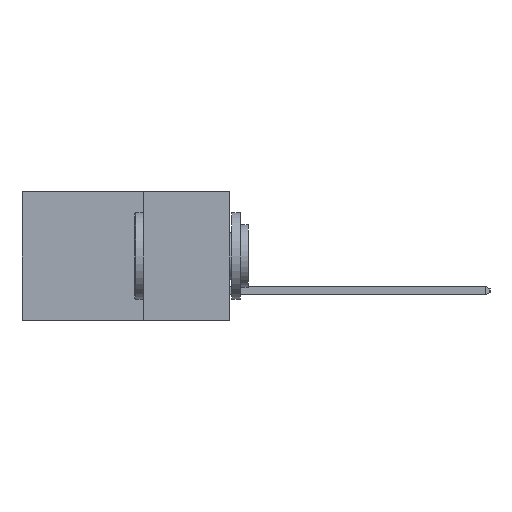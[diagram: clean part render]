
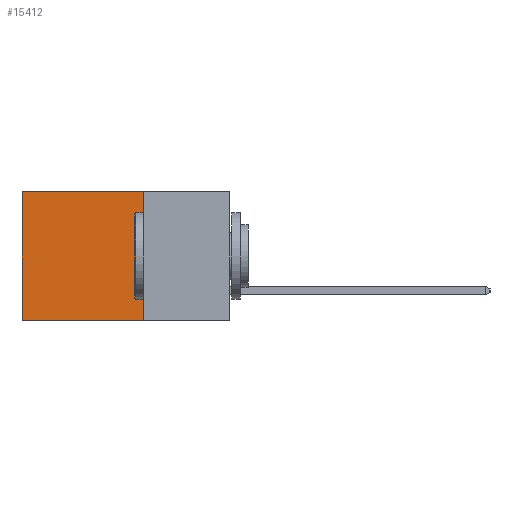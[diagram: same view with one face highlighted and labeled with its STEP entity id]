
A CAD part, left-side view. The second image highlights one B-rep face of the part: STEP entity #15412.
In plain terms, the highlighted planar face has unit normal (-1, 0, 0).
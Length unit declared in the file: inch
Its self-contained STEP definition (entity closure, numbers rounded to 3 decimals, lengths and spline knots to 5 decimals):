
#64 = VECTOR ( 'NONE', #19857, 39.37008 ) ;
#353 = DIRECTION ( 'NONE',  ( 0., 0., -1. ) ) ;
#356 = DIRECTION ( 'NONE',  ( 1., 0., 0. ) ) ;
#441 = PLANE ( 'NONE',  #8171 ) ;
#489 = CARTESIAN_POINT ( 'NONE',  ( 0.2615, 0.25, -0.37 ) ) ;
#1026 = ORIENTED_EDGE ( 'NONE', *, *, #11338, .T. ) ;
#1472 = LINE ( 'NONE', #2624, #6753 ) ;
#2441 = DIRECTION ( 'NONE',  ( 0., 0., -1. ) ) ;
#2473 = ORIENTED_EDGE ( 'NONE', *, *, #11125, .F. ) ;
#2490 = DIRECTION ( 'NONE',  ( 0., 1., 0. ) ) ;
#2624 = CARTESIAN_POINT ( 'NONE',  ( 0.2615, 0.6, -0.37 ) ) ;
#4432 = VERTEX_POINT ( 'NONE', #12737 ) ;
#5304 = EDGE_LOOP ( 'NONE', ( #17439, #21790, #2473, #1026 ) ) ;
#5968 = VERTEX_POINT ( 'NONE', #16197 ) ;
#6753 = VECTOR ( 'NONE', #2441, 39.37008 ) ;
#7382 = VERTEX_POINT ( 'NONE', #9404 ) ;
#8124 = CARTESIAN_POINT ( 'NONE',  ( 0.2615, 0.25, 0. ) ) ;
#8171 = AXIS2_PLACEMENT_3D ( 'NONE', #489, #356, #353 ) ;
#9142 = LINE ( 'NONE', #15837, #21863 ) ;
#9404 = CARTESIAN_POINT ( 'NONE',  ( 0.2615, 0.6, 0. ) ) ;
#10405 = EDGE_CURVE ( 'NONE', #7382, #5968, #1472, .T. ) ;
#11125 = EDGE_CURVE ( 'NONE', #13393, #4432, #13345, .T. ) ;
#11338 = EDGE_CURVE ( 'NONE', #13393, #7382, #9142, .T. ) ;
#12737 = CARTESIAN_POINT ( 'NONE',  ( 0.2615, 0.25, -0.37 ) ) ;
#12881 = CARTESIAN_POINT ( 'NONE',  ( 0.2615, 0.25, -0.37 ) ) ;
#13345 = LINE ( 'NONE', #20121, #64 ) ;
#13393 = VERTEX_POINT ( 'NONE', #8124 ) ;
#13576 = LINE ( 'NONE', #12881, #18036 ) ;
#15412 = ADVANCED_FACE ( 'NONE', ( #16818 ), #441, .F. ) ;
#15837 = CARTESIAN_POINT ( 'NONE',  ( 0.2615, 0.25, 0. ) ) ;
#16197 = CARTESIAN_POINT ( 'NONE',  ( 0.2615, 0.6, -0.37 ) ) ;
#16368 = DIRECTION ( 'NONE',  ( 0., 1., 0. ) ) ;
#16818 = FACE_OUTER_BOUND ( 'NONE', #5304, .T. ) ;
#17439 = ORIENTED_EDGE ( 'NONE', *, *, #10405, .T. ) ;
#18036 = VECTOR ( 'NONE', #2490, 39.37008 ) ;
#19857 = DIRECTION ( 'NONE',  ( 0., 0., -1. ) ) ;
#20121 = CARTESIAN_POINT ( 'NONE',  ( 0.2615, 0.25, -0.37 ) ) ;
#21790 = ORIENTED_EDGE ( 'NONE', *, *, #21913, .F. ) ;
#21863 = VECTOR ( 'NONE', #16368, 39.37008 ) ;
#21913 = EDGE_CURVE ( 'NONE', #4432, #5968, #13576, .T. ) ;
